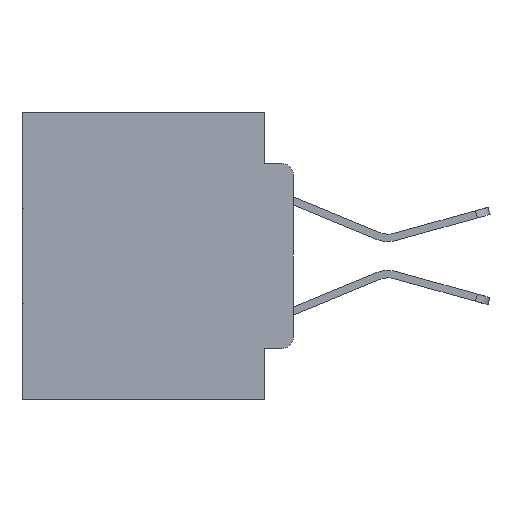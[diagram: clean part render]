
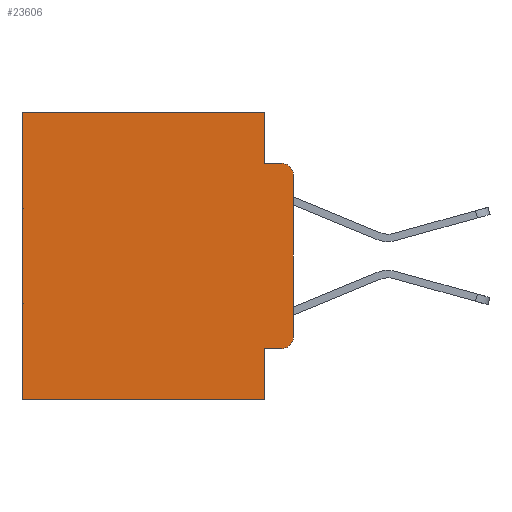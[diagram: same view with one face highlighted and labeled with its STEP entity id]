
A CAD part, left-side view. The second image highlights one B-rep face of the part: STEP entity #23606.
In plain terms, the highlighted planar face has unit normal (-1, 0, 0).
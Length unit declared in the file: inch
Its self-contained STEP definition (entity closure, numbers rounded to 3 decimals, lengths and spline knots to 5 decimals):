
#507 = ORIENTED_EDGE ( 'NONE', *, *, #19454, .T. ) ;
#732 = CARTESIAN_POINT ( 'NONE',  ( 0.298, 0.473, -0.5 ) ) ;
#1073 = AXIS2_PLACEMENT_3D ( 'NONE', #26157, #11861, #28489 ) ;
#1200 = CARTESIAN_POINT ( 'NONE',  ( 0.298, 0., 0. ) ) ;
#1456 = CARTESIAN_POINT ( 'NONE',  ( 0.298, 0., 0. ) ) ;
#1520 = CARTESIAN_POINT ( 'NONE',  ( 0.298, 0.02, -0.4115 ) ) ;
#1544 = VERTEX_POINT ( 'NONE', #732 ) ;
#1572 = EDGE_CURVE ( 'NONE', #28095, #7939, #3173, .T. ) ;
#1619 = VECTOR ( 'NONE', #21063, 39.37008 ) ;
#1781 = VECTOR ( 'NONE', #13466, 39.37008 ) ;
#2131 = ORIENTED_EDGE ( 'NONE', *, *, #25752, .F. ) ;
#2468 = VERTEX_POINT ( 'NONE', #2907 ) ;
#2566 = LINE ( 'NONE', #9934, #8448 ) ;
#2907 = CARTESIAN_POINT ( 'NONE',  ( 0.298, 0.02, -0.0885 ) ) ;
#3173 = LINE ( 'NONE', #1200, #28050 ) ;
#3482 = DIRECTION ( 'NONE',  ( 0., 1., 0. ) ) ;
#3529 = DIRECTION ( 'NONE',  ( 0., -1., 0. ) ) ;
#4136 = EDGE_CURVE ( 'NONE', #13500, #2468, #12259, .T. ) ;
#4209 = LINE ( 'NONE', #18347, #1781 ) ;
#4563 = ORIENTED_EDGE ( 'NONE', *, *, #27336, .T. ) ;
#4738 = CARTESIAN_POINT ( 'NONE',  ( 0.298, 0.051, -0.0885 ) ) ;
#4929 = CARTESIAN_POINT ( 'NONE',  ( 0.298, 0.051, -0.0885 ) ) ;
#5278 = CARTESIAN_POINT ( 'NONE',  ( 0.298, 0., -0.1085 ) ) ;
#5831 = EDGE_CURVE ( 'NONE', #21655, #2468, #23029, .T. ) ;
#6062 = DIRECTION ( 'NONE',  ( 0., 0., -1. ) ) ;
#7041 = VECTOR ( 'NONE', #3529, 39.37008 ) ;
#7198 = CARTESIAN_POINT ( 'NONE',  ( 0.298, 0., 0. ) ) ;
#7329 = CARTESIAN_POINT ( 'NONE',  ( 0.298, 0.051, -0.5 ) ) ;
#7939 = VERTEX_POINT ( 'NONE', #22468 ) ;
#8039 = ORIENTED_EDGE ( 'NONE', *, *, #21044, .T. ) ;
#8448 = VECTOR ( 'NONE', #17144, 39.37008 ) ;
#9765 = DIRECTION ( 'NONE',  ( 0., -1., 0. ) ) ;
#9934 = CARTESIAN_POINT ( 'NONE',  ( 0.298, 0., -0.5 ) ) ;
#10645 = CARTESIAN_POINT ( 'NONE',  ( 0.298, 0.02, -0.3915 ) ) ;
#11861 = DIRECTION ( 'NONE',  ( -1., 0., 0. ) ) ;
#11989 = LINE ( 'NONE', #14902, #7041 ) ;
#12259 = LINE ( 'NONE', #4929, #18711 ) ;
#13064 = DIRECTION ( 'NONE',  ( 0., 0., -1. ) ) ;
#13466 = DIRECTION ( 'NONE',  ( 0., 0., -1. ) ) ;
#13500 = VERTEX_POINT ( 'NONE', #4738 ) ;
#13554 = CARTESIAN_POINT ( 'NONE',  ( 0.298, 0., -0.3915 ) ) ;
#13722 = AXIS2_PLACEMENT_3D ( 'NONE', #10645, #27331, #13064 ) ;
#13985 = EDGE_CURVE ( 'NONE', #21655, #20216, #27410, .T. ) ;
#14527 = PLANE ( 'NONE',  #25178 ) ;
#14902 = CARTESIAN_POINT ( 'NONE',  ( 0.298, 0.051, -0.4115 ) ) ;
#15253 = ORIENTED_EDGE ( 'NONE', *, *, #26155, .F. ) ;
#16400 = ORIENTED_EDGE ( 'NONE', *, *, #28869, .F. ) ;
#16957 = DIRECTION ( 'NONE',  ( 0., 0., -1. ) ) ;
#17091 = DIRECTION ( 'NONE',  ( 0., 0., -1. ) ) ;
#17105 = VERTEX_POINT ( 'NONE', #1520 ) ;
#17144 = DIRECTION ( 'NONE',  ( 0., 1., 0. ) ) ;
#18347 = CARTESIAN_POINT ( 'NONE',  ( 0.298, 0.051, 0. ) ) ;
#18603 = VERTEX_POINT ( 'NONE', #19131 ) ;
#18609 = VECTOR ( 'NONE', #17091, 39.37008 ) ;
#18711 = VECTOR ( 'NONE', #9765, 39.37008 ) ;
#18876 = VECTOR ( 'NONE', #6062, 39.37008 ) ;
#19131 = CARTESIAN_POINT ( 'NONE',  ( 0.298, 0.051, -0.4115 ) ) ;
#19236 = VERTEX_POINT ( 'NONE', #7329 ) ;
#19454 = EDGE_CURVE ( 'NONE', #17105, #20216, #27408, .T. ) ;
#19630 = LINE ( 'NONE', #25292, #18876 ) ;
#20216 = VERTEX_POINT ( 'NONE', #13554 ) ;
#21044 = EDGE_CURVE ( 'NONE', #18603, #17105, #11989, .T. ) ;
#21063 = DIRECTION ( 'NONE',  ( 0., 0., -1. ) ) ;
#21655 = VERTEX_POINT ( 'NONE', #5278 ) ;
#22468 = CARTESIAN_POINT ( 'NONE',  ( 0.298, 0.473, 0. ) ) ;
#23029 = CIRCLE ( 'NONE', #1073, 0.02 ) ;
#23606 = ADVANCED_FACE ( 'NONE', ( #26756 ), #14527, .F. ) ;
#23825 = ORIENTED_EDGE ( 'NONE', *, *, #1572, .T. ) ;
#24872 = LINE ( 'NONE', #26498, #18609 ) ;
#25178 = AXIS2_PLACEMENT_3D ( 'NONE', #7198, #31107, #16957 ) ;
#25284 = ORIENTED_EDGE ( 'NONE', *, *, #5831, .T. ) ;
#25292 = CARTESIAN_POINT ( 'NONE',  ( 0.298, 0.051, 0. ) ) ;
#25752 = EDGE_CURVE ( 'NONE', #18603, #19236, #4209, .T. ) ;
#26018 = ORIENTED_EDGE ( 'NONE', *, *, #13985, .F. ) ;
#26155 = EDGE_CURVE ( 'NONE', #19236, #1544, #2566, .T. ) ;
#26157 = CARTESIAN_POINT ( 'NONE',  ( 0.298, 0.02, -0.1085 ) ) ;
#26498 = CARTESIAN_POINT ( 'NONE',  ( 0.298, 0.473, 0. ) ) ;
#26756 = FACE_OUTER_BOUND ( 'NONE', #30538, .T. ) ;
#27090 = CARTESIAN_POINT ( 'NONE',  ( 0.298, 0.051, 0. ) ) ;
#27331 = DIRECTION ( 'NONE',  ( -1., 0., 0. ) ) ;
#27336 = EDGE_CURVE ( 'NONE', #7939, #1544, #24872, .T. ) ;
#27408 = CIRCLE ( 'NONE', #13722, 0.02 ) ;
#27410 = LINE ( 'NONE', #1456, #1619 ) ;
#28050 = VECTOR ( 'NONE', #3482, 39.37008 ) ;
#28095 = VERTEX_POINT ( 'NONE', #27090 ) ;
#28489 = DIRECTION ( 'NONE',  ( 0., 0., -1. ) ) ;
#28869 = EDGE_CURVE ( 'NONE', #28095, #13500, #19630, .T. ) ;
#28966 = ORIENTED_EDGE ( 'NONE', *, *, #4136, .F. ) ;
#30538 = EDGE_LOOP ( 'NONE', ( #26018, #25284, #28966, #16400, #23825, #4563, #15253, #2131, #8039, #507 ) ) ;
#31107 = DIRECTION ( 'NONE',  ( 1., 0., 0. ) ) ;
